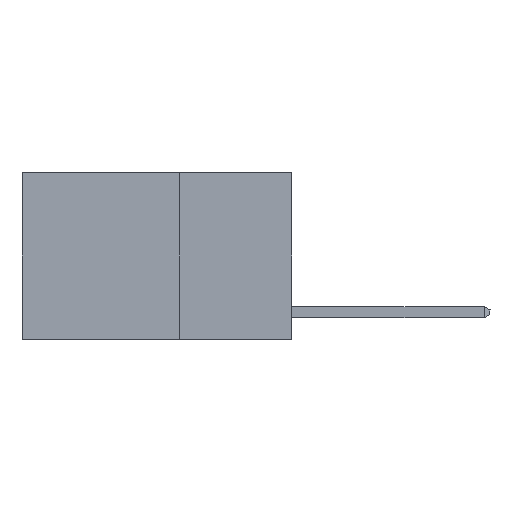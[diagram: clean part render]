
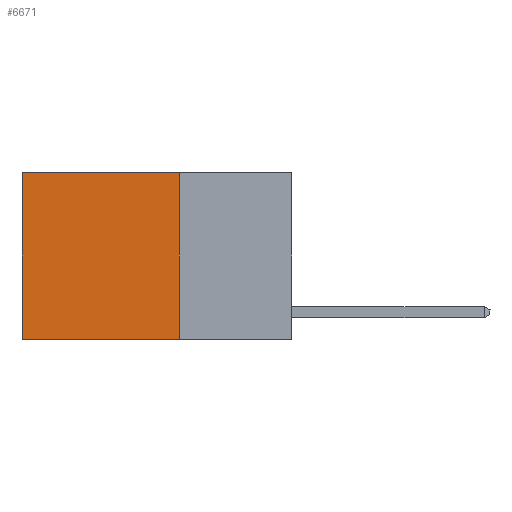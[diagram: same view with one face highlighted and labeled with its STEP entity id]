
A CAD part, left-side view. The second image highlights one B-rep face of the part: STEP entity #6671.
In plain terms, the highlighted planar face has unit normal (-1, 0, 0).
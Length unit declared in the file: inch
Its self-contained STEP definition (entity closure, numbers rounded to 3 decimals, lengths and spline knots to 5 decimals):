
#120 = VERTEX_POINT ( 'NONE', #7285 ) ;
#193 = VERTEX_POINT ( 'NONE', #9845 ) ;
#668 = VECTOR ( 'NONE', #4412, 39.37008 ) ;
#719 = VERTEX_POINT ( 'NONE', #14333 ) ;
#852 = VECTOR ( 'NONE', #8509, 39.37008 ) ;
#1062 = LINE ( 'NONE', #5541, #668 ) ;
#1189 = PLANE ( 'NONE',  #3012 ) ;
#1670 = ORIENTED_EDGE ( 'NONE', *, *, #11249, .F. ) ;
#1949 = CARTESIAN_POINT ( 'NONE',  ( 0.2625, 0.6, 0. ) ) ;
#2405 = DIRECTION ( 'NONE',  ( 0., 0., -1. ) ) ;
#3012 = AXIS2_PLACEMENT_3D ( 'NONE', #14394, #9721, #2405 ) ;
#3394 = ORIENTED_EDGE ( 'NONE', *, *, #14482, .T. ) ;
#4081 = LINE ( 'NONE', #10857, #852 ) ;
#4412 = DIRECTION ( 'NONE',  ( 0., 0., -1. ) ) ;
#4558 = EDGE_LOOP ( 'NONE', ( #10375, #5657, #1670, #3394 ) ) ;
#4948 = FACE_OUTER_BOUND ( 'NONE', #4558, .T. ) ;
#5541 = CARTESIAN_POINT ( 'NONE',  ( 0.2625, 0.6, 0. ) ) ;
#5657 = ORIENTED_EDGE ( 'NONE', *, *, #15209, .F. ) ;
#6671 = ADVANCED_FACE ( 'NONE', ( #4948 ), #1189, .F. ) ;
#7217 = DIRECTION ( 'NONE',  ( 0., 0., -1. ) ) ;
#7285 = CARTESIAN_POINT ( 'NONE',  ( 0.2625, 0.6, -0.37 ) ) ;
#7727 = VERTEX_POINT ( 'NONE', #1949 ) ;
#8093 = DIRECTION ( 'NONE',  ( 0., 1., 0. ) ) ;
#8447 = CARTESIAN_POINT ( 'NONE',  ( 0.2625, 0.25, 0. ) ) ;
#8509 = DIRECTION ( 'NONE',  ( 0., 1., 0. ) ) ;
#9721 = DIRECTION ( 'NONE',  ( 1., 0., 0. ) ) ;
#9845 = CARTESIAN_POINT ( 'NONE',  ( 0.2625, 0.25, -0.37 ) ) ;
#10375 = ORIENTED_EDGE ( 'NONE', *, *, #13164, .T. ) ;
#10857 = CARTESIAN_POINT ( 'NONE',  ( 0.2625, 0.25, -0.37 ) ) ;
#11249 = EDGE_CURVE ( 'NONE', #719, #193, #13762, .T. ) ;
#11461 = LINE ( 'NONE', #12829, #14965 ) ;
#12829 = CARTESIAN_POINT ( 'NONE',  ( 0.2625, 0.25, 0. ) ) ;
#13164 = EDGE_CURVE ( 'NONE', #7727, #120, #1062, .T. ) ;
#13408 = VECTOR ( 'NONE', #7217, 39.37008 ) ;
#13762 = LINE ( 'NONE', #8447, #13408 ) ;
#14333 = CARTESIAN_POINT ( 'NONE',  ( 0.2625, 0.25, 0. ) ) ;
#14394 = CARTESIAN_POINT ( 'NONE',  ( 0.2625, 0.25, 0. ) ) ;
#14482 = EDGE_CURVE ( 'NONE', #719, #7727, #11461, .T. ) ;
#14965 = VECTOR ( 'NONE', #8093, 39.37008 ) ;
#15209 = EDGE_CURVE ( 'NONE', #193, #120, #4081, .T. ) ;
